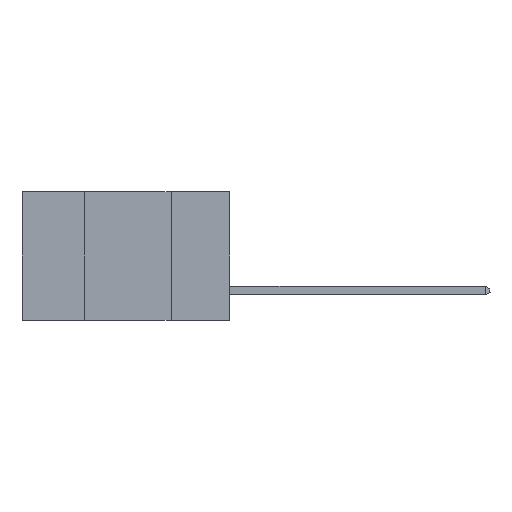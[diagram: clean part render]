
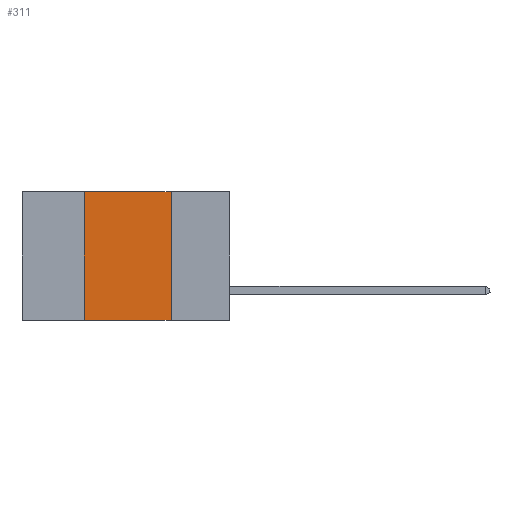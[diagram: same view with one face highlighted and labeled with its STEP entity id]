
A CAD part, left-side view. The second image highlights one B-rep face of the part: STEP entity #311.
In plain terms, the highlighted planar face has unit normal (-1, 0, 0).
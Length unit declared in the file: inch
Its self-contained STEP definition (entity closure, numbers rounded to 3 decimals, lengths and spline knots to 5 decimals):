
#79 = LINE ( 'NONE', #951, #4132 ) ;
#192 = VECTOR ( 'NONE', #1275, 39.37008 ) ;
#311 = ADVANCED_FACE ( 'NONE', ( #6285 ), #835, .F. ) ;
#835 = PLANE ( 'NONE',  #4006 ) ;
#951 = CARTESIAN_POINT ( 'NONE',  ( 0., 0.42, 0. ) ) ;
#1275 = DIRECTION ( 'NONE',  ( 0., 0., -1. ) ) ;
#1390 = DIRECTION ( 'NONE',  ( 0., 0., 1. ) ) ;
#1622 = VECTOR ( 'NONE', #4362, 39.37008 ) ;
#1772 = EDGE_CURVE ( 'NONE', #2378, #1811, #8611, .T. ) ;
#1811 = VERTEX_POINT ( 'NONE', #6887 ) ;
#1950 = LINE ( 'NONE', #3318, #3750 ) ;
#2076 = CARTESIAN_POINT ( 'NONE',  ( 0., 0.42, -0.37 ) ) ;
#2378 = VERTEX_POINT ( 'NONE', #2076 ) ;
#2712 = EDGE_LOOP ( 'NONE', ( #3968, #3974, #3881, #3916 ) ) ;
#2740 = VERTEX_POINT ( 'NONE', #3919 ) ;
#2799 = DIRECTION ( 'NONE',  ( 1., 0., 0. ) ) ;
#2812 = DIRECTION ( 'NONE',  ( 0., 0., -1. ) ) ;
#3296 = EDGE_CURVE ( 'NONE', #2378, #2740, #79, .T. ) ;
#3318 = CARTESIAN_POINT ( 'NONE',  ( 0., 0.6, 0. ) ) ;
#3561 = EDGE_CURVE ( 'NONE', #2740, #6735, #1950, .T. ) ;
#3750 = VECTOR ( 'NONE', #6376, 39.37008 ) ;
#3758 = CARTESIAN_POINT ( 'NONE',  ( 0., 0.17, 0. ) ) ;
#3881 = ORIENTED_EDGE ( 'NONE', *, *, #3296, .F. ) ;
#3916 = ORIENTED_EDGE ( 'NONE', *, *, #1772, .T. ) ;
#3919 = CARTESIAN_POINT ( 'NONE',  ( 0., 0.42, 0. ) ) ;
#3968 = ORIENTED_EDGE ( 'NONE', *, *, #4354, .F. ) ;
#3974 = ORIENTED_EDGE ( 'NONE', *, *, #3561, .F. ) ;
#4006 = AXIS2_PLACEMENT_3D ( 'NONE', #8376, #2799, #2812 ) ;
#4132 = VECTOR ( 'NONE', #1390, 39.37008 ) ;
#4266 = CARTESIAN_POINT ( 'NONE',  ( 0., 0.6, -0.37 ) ) ;
#4354 = EDGE_CURVE ( 'NONE', #6735, #1811, #5952, .T. ) ;
#4362 = DIRECTION ( 'NONE',  ( 0., -1., 0. ) ) ;
#5952 = LINE ( 'NONE', #6296, #192 ) ;
#6285 = FACE_OUTER_BOUND ( 'NONE', #2712, .T. ) ;
#6296 = CARTESIAN_POINT ( 'NONE',  ( 0., 0.17, 0. ) ) ;
#6376 = DIRECTION ( 'NONE',  ( 0., -1., 0. ) ) ;
#6735 = VERTEX_POINT ( 'NONE', #3758 ) ;
#6887 = CARTESIAN_POINT ( 'NONE',  ( 0., 0.17, -0.37 ) ) ;
#8376 = CARTESIAN_POINT ( 'NONE',  ( 0., 0.6, 0. ) ) ;
#8611 = LINE ( 'NONE', #4266, #1622 ) ;
